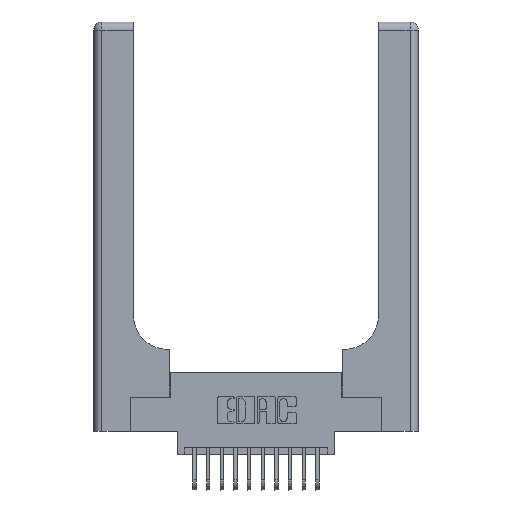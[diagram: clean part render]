
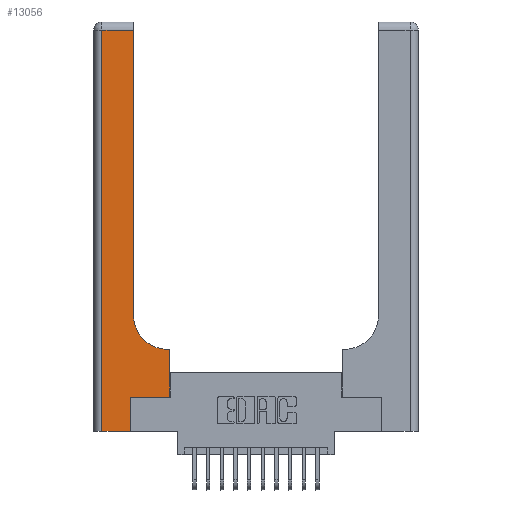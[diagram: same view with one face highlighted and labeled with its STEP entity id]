
A CAD part, top view. The second image highlights one B-rep face of the part: STEP entity #13056.
In plain terms, the highlighted planar face has unit normal (0, 0, 1).
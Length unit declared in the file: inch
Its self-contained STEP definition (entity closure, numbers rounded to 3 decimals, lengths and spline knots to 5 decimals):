
#198 = ORIENTED_EDGE ( 'NONE', *, *, #14572, .T. ) ;
#291 = VERTEX_POINT ( 'NONE', #11606 ) ;
#525 = CARTESIAN_POINT ( 'NONE',  ( 0.5415, 0.6, 0.37 ) ) ;
#538 = DIRECTION ( 'NONE',  ( -1., 0., 0. ) ) ;
#556 = EDGE_CURVE ( 'NONE', #17764, #4761, #7894, .T. ) ;
#761 = CARTESIAN_POINT ( 'NONE',  ( 0.269, 0., 0.37 ) ) ;
#1012 = CARTESIAN_POINT ( 'NONE',  ( 0.2915, 2.94, 0.37 ) ) ;
#1029 = LINE ( 'NONE', #15353, #6786 ) ;
#1361 = EDGE_CURVE ( 'NONE', #6581, #13555, #5539, .T. ) ;
#1456 = ORIENTED_EDGE ( 'NONE', *, *, #14772, .T. ) ;
#2347 = LINE ( 'NONE', #11613, #9946 ) ;
#2566 = DIRECTION ( 'NONE',  ( 1., 0., 0. ) ) ;
#2938 = EDGE_CURVE ( 'NONE', #6232, #9833, #9196, .T. ) ;
#3474 = DIRECTION ( 'NONE',  ( 1., 0., 0. ) ) ;
#3487 = VERTEX_POINT ( 'NONE', #1012 ) ;
#3615 = DIRECTION ( 'NONE',  ( 1., 0., 0. ) ) ;
#3682 = DIRECTION ( 'NONE',  ( 0., 0., -1. ) ) ;
#3813 = CARTESIAN_POINT ( 'NONE',  ( 0.06, 0., 0.37 ) ) ;
#4104 = CARTESIAN_POINT ( 'NONE',  ( 0.06, 3., 0.37 ) ) ;
#4162 = ORIENTED_EDGE ( 'NONE', *, *, #8502, .T. ) ;
#4443 = FACE_OUTER_BOUND ( 'NONE', #11325, .T. ) ;
#4655 = ORIENTED_EDGE ( 'NONE', *, *, #17644, .T. ) ;
#4761 = VERTEX_POINT ( 'NONE', #16614 ) ;
#5336 = CARTESIAN_POINT ( 'NONE',  ( 0., 3., 0.37 ) ) ;
#5539 = LINE ( 'NONE', #9353, #16464 ) ;
#5852 = ORIENTED_EDGE ( 'NONE', *, *, #9478, .T. ) ;
#6232 = VERTEX_POINT ( 'NONE', #14556 ) ;
#6349 = LINE ( 'NONE', #17594, #10291 ) ;
#6525 = CARTESIAN_POINT ( 'NONE',  ( 0.269, 0.25, 0.37 ) ) ;
#6581 = VERTEX_POINT ( 'NONE', #761 ) ;
#6786 = VECTOR ( 'NONE', #12230, 39.37008 ) ;
#6828 = VERTEX_POINT ( 'NONE', #7489 ) ;
#7489 = CARTESIAN_POINT ( 'NONE',  ( 0.5585, 0.25, 0.37 ) ) ;
#7856 = DIRECTION ( 'NONE',  ( 0., 1., 0. ) ) ;
#7894 = CIRCLE ( 'NONE', #10048, 0.25 ) ;
#8502 = EDGE_CURVE ( 'NONE', #6828, #291, #6349, .T. ) ;
#9196 = LINE ( 'NONE', #4104, #16166 ) ;
#9220 = DIRECTION ( 'NONE',  ( -1., 0., 0. ) ) ;
#9353 = CARTESIAN_POINT ( 'NONE',  ( 0.269, 0., 0.37 ) ) ;
#9478 = EDGE_CURVE ( 'NONE', #4761, #3487, #1029, .T. ) ;
#9606 = DIRECTION ( 'NONE',  ( 0., 0., -1. ) ) ;
#9833 = VERTEX_POINT ( 'NONE', #3813 ) ;
#9946 = VECTOR ( 'NONE', #2566, 39.37008 ) ;
#10048 = AXIS2_PLACEMENT_3D ( 'NONE', #13788, #9606, #3615 ) ;
#10291 = VECTOR ( 'NONE', #13134, 39.37008 ) ;
#11325 = EDGE_LOOP ( 'NONE', ( #5852, #4655, #17563, #1456, #18637, #198, #4162, #18687, #16018 ) ) ;
#11409 = VECTOR ( 'NONE', #538, 39.37008 ) ;
#11606 = CARTESIAN_POINT ( 'NONE',  ( 0.5585, 0.6, 0.37 ) ) ;
#11613 = CARTESIAN_POINT ( 'NONE',  ( 0., 0., 0.37 ) ) ;
#12087 = CARTESIAN_POINT ( 'NONE',  ( 0., 2.94, 0.37 ) ) ;
#12173 = CARTESIAN_POINT ( 'NONE',  ( 0.2915, 0.6, 0.37 ) ) ;
#12203 = EDGE_CURVE ( 'NONE', #291, #17764, #12604, .T. ) ;
#12230 = DIRECTION ( 'NONE',  ( 0., 1., 0. ) ) ;
#12304 = VECTOR ( 'NONE', #3474, 39.37008 ) ;
#12358 = CARTESIAN_POINT ( 'NONE',  ( 0.269, 0.25, 0.37 ) ) ;
#12604 = LINE ( 'NONE', #12173, #11409 ) ;
#12739 = DIRECTION ( 'NONE',  ( -1., 0., 0. ) ) ;
#13056 = ADVANCED_FACE ( 'NONE', ( #4443 ), #18554, .F. ) ;
#13134 = DIRECTION ( 'NONE',  ( 0., 1., 0. ) ) ;
#13555 = VERTEX_POINT ( 'NONE', #6525 ) ;
#13788 = CARTESIAN_POINT ( 'NONE',  ( 0.5415, 0.85, 0.37 ) ) ;
#14556 = CARTESIAN_POINT ( 'NONE',  ( 0.06, 2.94, 0.37 ) ) ;
#14572 = EDGE_CURVE ( 'NONE', #13555, #6828, #18760, .T. ) ;
#14772 = EDGE_CURVE ( 'NONE', #9833, #6581, #2347, .T. ) ;
#15353 = CARTESIAN_POINT ( 'NONE',  ( 0.2915, 3., 0.37 ) ) ;
#16018 = ORIENTED_EDGE ( 'NONE', *, *, #556, .T. ) ;
#16166 = VECTOR ( 'NONE', #17977, 39.37008 ) ;
#16464 = VECTOR ( 'NONE', #7856, 39.37008 ) ;
#16614 = CARTESIAN_POINT ( 'NONE',  ( 0.2915, 0.85, 0.37 ) ) ;
#17066 = LINE ( 'NONE', #12087, #18651 ) ;
#17180 = AXIS2_PLACEMENT_3D ( 'NONE', #5336, #3682, #12739 ) ;
#17563 = ORIENTED_EDGE ( 'NONE', *, *, #2938, .T. ) ;
#17594 = CARTESIAN_POINT ( 'NONE',  ( 0.5585, 0.25, 0.37 ) ) ;
#17644 = EDGE_CURVE ( 'NONE', #3487, #6232, #17066, .T. ) ;
#17764 = VERTEX_POINT ( 'NONE', #525 ) ;
#17977 = DIRECTION ( 'NONE',  ( 0., -1., 0. ) ) ;
#18554 = PLANE ( 'NONE',  #17180 ) ;
#18637 = ORIENTED_EDGE ( 'NONE', *, *, #1361, .T. ) ;
#18651 = VECTOR ( 'NONE', #9220, 39.37008 ) ;
#18687 = ORIENTED_EDGE ( 'NONE', *, *, #12203, .T. ) ;
#18760 = LINE ( 'NONE', #12358, #12304 ) ;
